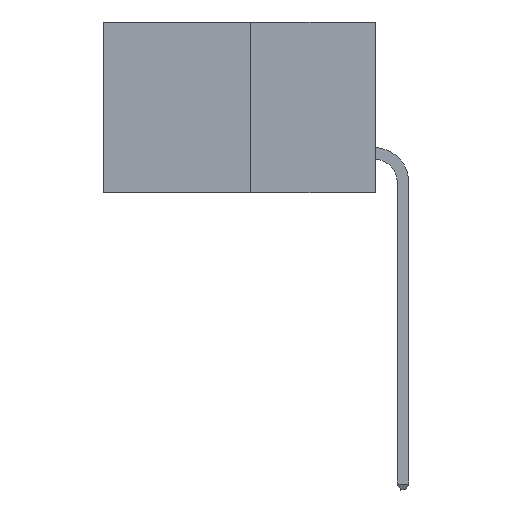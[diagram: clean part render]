
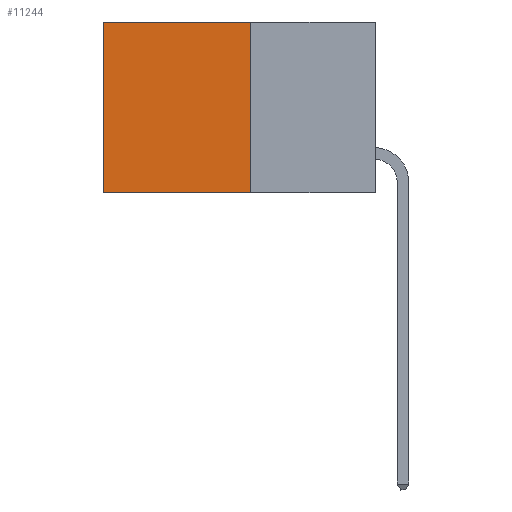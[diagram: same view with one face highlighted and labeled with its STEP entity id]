
A CAD part, left-side view. The second image highlights one B-rep face of the part: STEP entity #11244.
In plain terms, the highlighted planar face has unit normal (-1, 0, 0).
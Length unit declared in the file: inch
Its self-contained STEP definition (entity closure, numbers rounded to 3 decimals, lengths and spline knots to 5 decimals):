
#6 = DIRECTION ( 'NONE',  ( 0., 0., -1. ) ) ;
#71 = EDGE_CURVE ( 'NONE', #12762, #4438, #12746, .T. ) ;
#157 = CARTESIAN_POINT ( 'NONE',  ( 0.277, 0.27, -0.37 ) ) ;
#233 = DIRECTION ( 'NONE',  ( 0., 0., -1. ) ) ;
#457 = CARTESIAN_POINT ( 'NONE',  ( 0.277, 0.27, -0.37 ) ) ;
#2595 = EDGE_CURVE ( 'NONE', #12594, #12762, #11208, .T. ) ;
#3219 = CARTESIAN_POINT ( 'NONE',  ( 0.277, 0.27, 0. ) ) ;
#3659 = EDGE_LOOP ( 'NONE', ( #17164, #6646, #10036, #4986 ) ) ;
#4047 = CARTESIAN_POINT ( 'NONE',  ( 0.277, 0.27, -0.37 ) ) ;
#4224 = EDGE_CURVE ( 'NONE', #17026, #4438, #4845, .T. ) ;
#4438 = VERTEX_POINT ( 'NONE', #7757 ) ;
#4845 = LINE ( 'NONE', #12682, #7586 ) ;
#4986 = ORIENTED_EDGE ( 'NONE', *, *, #10205, .T. ) ;
#5435 = DIRECTION ( 'NONE',  ( 0., 1., 0. ) ) ;
#5475 = CARTESIAN_POINT ( 'NONE',  ( 0.277, 0.59, 0. ) ) ;
#5540 = PLANE ( 'NONE',  #7483 ) ;
#6646 = ORIENTED_EDGE ( 'NONE', *, *, #71, .F. ) ;
#6861 = CARTESIAN_POINT ( 'NONE',  ( 0.277, 0.27, -0.37 ) ) ;
#7483 = AXIS2_PLACEMENT_3D ( 'NONE', #6861, #8199, #233 ) ;
#7586 = VECTOR ( 'NONE', #12826, 39.37008 ) ;
#7757 = CARTESIAN_POINT ( 'NONE',  ( 0.277, 0.59, -0.37 ) ) ;
#8199 = DIRECTION ( 'NONE',  ( 1., 0., 0. ) ) ;
#9197 = VECTOR ( 'NONE', #5435, 39.37008 ) ;
#9587 = VECTOR ( 'NONE', #12524, 39.37008 ) ;
#10036 = ORIENTED_EDGE ( 'NONE', *, *, #2595, .F. ) ;
#10205 = EDGE_CURVE ( 'NONE', #12594, #17026, #10425, .T. ) ;
#10425 = LINE ( 'NONE', #3219, #9587 ) ;
#11208 = LINE ( 'NONE', #157, #16551 ) ;
#11244 = ADVANCED_FACE ( 'NONE', ( #13260 ), #5540, .F. ) ;
#12524 = DIRECTION ( 'NONE',  ( 0., 1., 0. ) ) ;
#12594 = VERTEX_POINT ( 'NONE', #16736 ) ;
#12682 = CARTESIAN_POINT ( 'NONE',  ( 0.277, 0.59, -0.37 ) ) ;
#12746 = LINE ( 'NONE', #457, #9197 ) ;
#12762 = VERTEX_POINT ( 'NONE', #4047 ) ;
#12826 = DIRECTION ( 'NONE',  ( 0., 0., -1. ) ) ;
#13260 = FACE_OUTER_BOUND ( 'NONE', #3659, .T. ) ;
#16551 = VECTOR ( 'NONE', #6, 39.37008 ) ;
#16736 = CARTESIAN_POINT ( 'NONE',  ( 0.277, 0.27, 0. ) ) ;
#17026 = VERTEX_POINT ( 'NONE', #5475 ) ;
#17164 = ORIENTED_EDGE ( 'NONE', *, *, #4224, .T. ) ;
